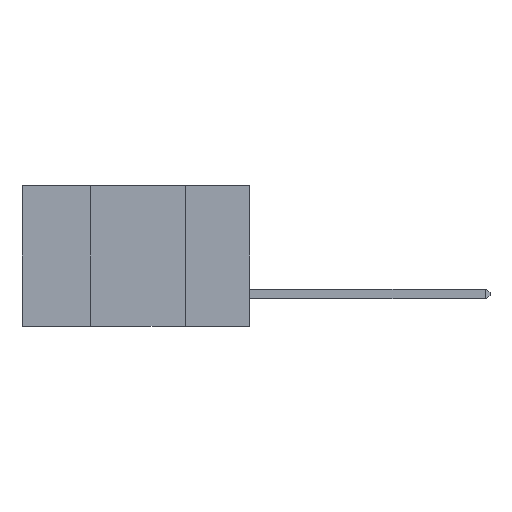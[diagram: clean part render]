
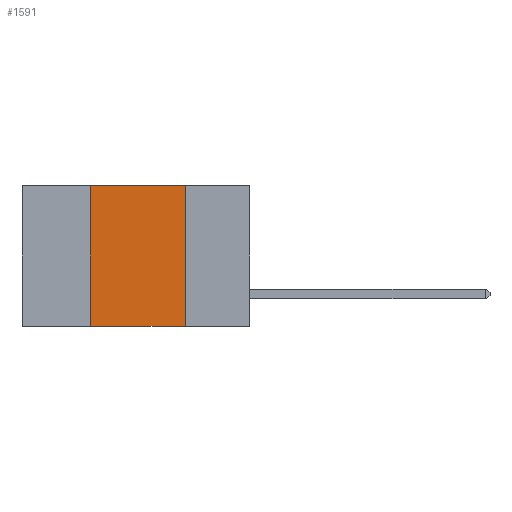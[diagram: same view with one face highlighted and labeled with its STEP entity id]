
A CAD part, left-side view. The second image highlights one B-rep face of the part: STEP entity #1591.
In plain terms, the highlighted planar face has unit normal (-1, 0, 0).
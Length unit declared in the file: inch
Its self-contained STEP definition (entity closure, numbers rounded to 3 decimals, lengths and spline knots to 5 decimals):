
#1458 = EDGE_CURVE ( 'NONE', #6027, #5030, #2638, .T. ) ;
#1517 = CARTESIAN_POINT ( 'NONE',  ( 0., 0.6, -0.37 ) ) ;
#1550 = DIRECTION ( 'NONE',  ( 0., -1., 0. ) ) ;
#1591 = ADVANCED_FACE ( 'NONE', ( #8876 ), #12579, .F. ) ;
#2183 = CARTESIAN_POINT ( 'NONE',  ( 0., 0.17, 0. ) ) ;
#2242 = CARTESIAN_POINT ( 'NONE',  ( 0., 0.17, -0.37 ) ) ;
#2434 = LINE ( 'NONE', #2183, #4855 ) ;
#2638 = LINE ( 'NONE', #12536, #10408 ) ;
#2834 = ORIENTED_EDGE ( 'NONE', *, *, #3590, .T. ) ;
#3239 = ORIENTED_EDGE ( 'NONE', *, *, #1458, .F. ) ;
#3508 = CARTESIAN_POINT ( 'NONE',  ( 0., 0.42, -0.37 ) ) ;
#3590 = EDGE_CURVE ( 'NONE', #6027, #11091, #8326, .T. ) ;
#4716 = EDGE_CURVE ( 'NONE', #5030, #5580, #6217, .T. ) ;
#4855 = VECTOR ( 'NONE', #6268, 39.37008 ) ;
#5030 = VERTEX_POINT ( 'NONE', #9925 ) ;
#5580 = VERTEX_POINT ( 'NONE', #6354 ) ;
#5909 = VECTOR ( 'NONE', #11821, 39.37008 ) ;
#6027 = VERTEX_POINT ( 'NONE', #3508 ) ;
#6217 = LINE ( 'NONE', #11797, #5909 ) ;
#6268 = DIRECTION ( 'NONE',  ( 0., 0., -1. ) ) ;
#6354 = CARTESIAN_POINT ( 'NONE',  ( 0., 0.17, 0. ) ) ;
#7904 = DIRECTION ( 'NONE',  ( 0., 0., 1. ) ) ;
#8284 = EDGE_LOOP ( 'NONE', ( #8670, #11614, #3239, #2834 ) ) ;
#8326 = LINE ( 'NONE', #1517, #10653 ) ;
#8670 = ORIENTED_EDGE ( 'NONE', *, *, #11680, .F. ) ;
#8876 = FACE_OUTER_BOUND ( 'NONE', #8284, .T. ) ;
#9588 = DIRECTION ( 'NONE',  ( 0., 0., -1. ) ) ;
#9641 = DIRECTION ( 'NONE',  ( 1., 0., 0. ) ) ;
#9925 = CARTESIAN_POINT ( 'NONE',  ( 0., 0.42, 0. ) ) ;
#10408 = VECTOR ( 'NONE', #7904, 39.37008 ) ;
#10653 = VECTOR ( 'NONE', #1550, 39.37008 ) ;
#11091 = VERTEX_POINT ( 'NONE', #2242 ) ;
#11614 = ORIENTED_EDGE ( 'NONE', *, *, #4716, .F. ) ;
#11680 = EDGE_CURVE ( 'NONE', #5580, #11091, #2434, .T. ) ;
#11797 = CARTESIAN_POINT ( 'NONE',  ( 0., 0.6, 0. ) ) ;
#11821 = DIRECTION ( 'NONE',  ( 0., -1., 0. ) ) ;
#11922 = AXIS2_PLACEMENT_3D ( 'NONE', #12559, #9641, #9588 ) ;
#12536 = CARTESIAN_POINT ( 'NONE',  ( 0., 0.42, 0. ) ) ;
#12559 = CARTESIAN_POINT ( 'NONE',  ( 0., 0.6, 0. ) ) ;
#12579 = PLANE ( 'NONE',  #11922 ) ;
